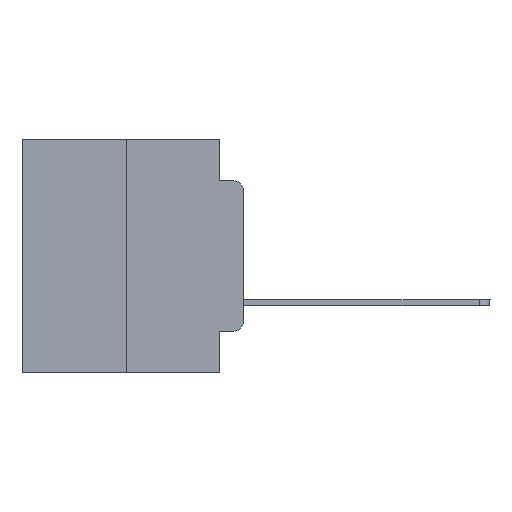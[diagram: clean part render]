
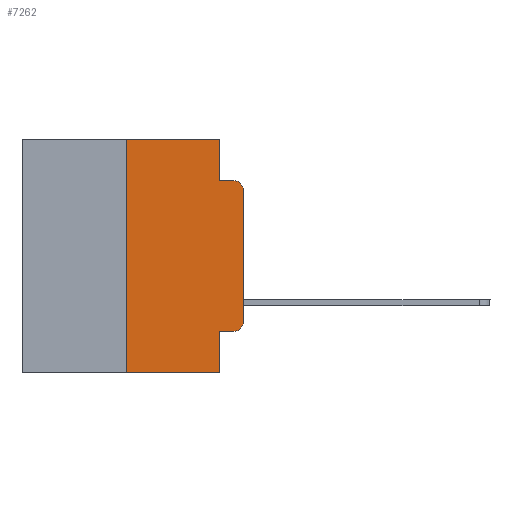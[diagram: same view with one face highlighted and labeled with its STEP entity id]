
A CAD part, left-side view. The second image highlights one B-rep face of the part: STEP entity #7262.
In plain terms, the highlighted planar face has unit normal (-1, 0, 0).
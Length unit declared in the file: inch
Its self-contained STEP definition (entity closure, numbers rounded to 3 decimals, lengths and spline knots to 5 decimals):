
#54 = LINE ( 'NONE', #8005, #21937 ) ;
#151 = CARTESIAN_POINT ( 'NONE',  ( 0., 0.02, -0.4115 ) ) ;
#272 = LINE ( 'NONE', #13980, #5402 ) ;
#963 = EDGE_CURVE ( 'NONE', #24113, #17036, #7960, .T. ) ;
#1355 = FACE_OUTER_BOUND ( 'NONE', #11826, .T. ) ;
#1591 = CARTESIAN_POINT ( 'NONE',  ( 0., 0.02, -0.0885 ) ) ;
#1706 = VECTOR ( 'NONE', #5119, 39.37008 ) ;
#1887 = CARTESIAN_POINT ( 'NONE',  ( 0., 0.25, 0. ) ) ;
#2122 = AXIS2_PLACEMENT_3D ( 'NONE', #11537, #19460, #17276 ) ;
#2824 = EDGE_CURVE ( 'NONE', #17036, #20742, #11524, .T. ) ;
#2998 = DIRECTION ( 'NONE',  ( 0., 0., -1. ) ) ;
#3121 = CARTESIAN_POINT ( 'NONE',  ( 0., 0.051, 0. ) ) ;
#3213 = VERTEX_POINT ( 'NONE', #18756 ) ;
#3263 = VERTEX_POINT ( 'NONE', #11593 ) ;
#3569 = PLANE ( 'NONE',  #2122 ) ;
#3600 = AXIS2_PLACEMENT_3D ( 'NONE', #15680, #3909, #11621 ) ;
#3909 = DIRECTION ( 'NONE',  ( -1., 0., 0. ) ) ;
#4227 = DIRECTION ( 'NONE',  ( 0., 0., -1. ) ) ;
#4660 = ORIENTED_EDGE ( 'NONE', *, *, #24435, .F. ) ;
#4749 = LINE ( 'NONE', #20508, #1706 ) ;
#4860 = ORIENTED_EDGE ( 'NONE', *, *, #963, .T. ) ;
#5119 = DIRECTION ( 'NONE',  ( 0., -1., 0. ) ) ;
#5402 = VECTOR ( 'NONE', #21869, 39.37008 ) ;
#5819 = EDGE_CURVE ( 'NONE', #13149, #12409, #4749, .T. ) ;
#6315 = ORIENTED_EDGE ( 'NONE', *, *, #11734, .F. ) ;
#6519 = EDGE_CURVE ( 'NONE', #13149, #14056, #272, .T. ) ;
#6989 = CARTESIAN_POINT ( 'NONE',  ( 0., 0.051, -0.0885 ) ) ;
#7262 = ADVANCED_FACE ( 'NONE', ( #1355 ), #3569, .F. ) ;
#7497 = ORIENTED_EDGE ( 'NONE', *, *, #25428, .T. ) ;
#7960 = LINE ( 'NONE', #9929, #23272 ) ;
#8005 = CARTESIAN_POINT ( 'NONE',  ( 0., 0., 0. ) ) ;
#8310 = ORIENTED_EDGE ( 'NONE', *, *, #6519, .F. ) ;
#8533 = CIRCLE ( 'NONE', #21038, 0.02 ) ;
#9397 = CARTESIAN_POINT ( 'NONE',  ( 0., 0.25, -0.5 ) ) ;
#9672 = DIRECTION ( 'NONE',  ( 0., 0., -1. ) ) ;
#9699 = VECTOR ( 'NONE', #24784, 39.37008 ) ;
#9929 = CARTESIAN_POINT ( 'NONE',  ( 0., 0.051, -0.4115 ) ) ;
#9946 = CARTESIAN_POINT ( 'NONE',  ( 0., 0., -0.1085 ) ) ;
#11093 = LINE ( 'NONE', #3121, #19722 ) ;
#11372 = VERTEX_POINT ( 'NONE', #1591 ) ;
#11524 = CIRCLE ( 'NONE', #3600, 0.02 ) ;
#11537 = CARTESIAN_POINT ( 'NONE',  ( 0., 0.473, 0. ) ) ;
#11593 = CARTESIAN_POINT ( 'NONE',  ( 0., 0.051, -0.0885 ) ) ;
#11621 = DIRECTION ( 'NONE',  ( 0., 0., -1. ) ) ;
#11689 = CARTESIAN_POINT ( 'NONE',  ( 0., 0.02, -0.1085 ) ) ;
#11734 = EDGE_CURVE ( 'NONE', #3213, #3263, #11093, .T. ) ;
#11826 = EDGE_LOOP ( 'NONE', ( #12894, #7497, #13380, #6315, #18050, #8310, #15507, #4660, #4860, #23856 ) ) ;
#11894 = VECTOR ( 'NONE', #22389, 39.37008 ) ;
#12409 = VERTEX_POINT ( 'NONE', #19884 ) ;
#12867 = EDGE_CURVE ( 'NONE', #14056, #3213, #24199, .T. ) ;
#12894 = ORIENTED_EDGE ( 'NONE', *, *, #15454, .T. ) ;
#13149 = VERTEX_POINT ( 'NONE', #9397 ) ;
#13380 = ORIENTED_EDGE ( 'NONE', *, *, #22109, .F. ) ;
#13848 = CARTESIAN_POINT ( 'NONE',  ( 0., 0.051, 0. ) ) ;
#13980 = CARTESIAN_POINT ( 'NONE',  ( 0., 0.25, 0. ) ) ;
#14056 = VERTEX_POINT ( 'NONE', #1887 ) ;
#14637 = CARTESIAN_POINT ( 'NONE',  ( 0., 0.473, 0. ) ) ;
#15454 = EDGE_CURVE ( 'NONE', #20742, #15766, #54, .T. ) ;
#15507 = ORIENTED_EDGE ( 'NONE', *, *, #5819, .T. ) ;
#15680 = CARTESIAN_POINT ( 'NONE',  ( 0., 0.02, -0.3915 ) ) ;
#15766 = VERTEX_POINT ( 'NONE', #9946 ) ;
#15978 = DIRECTION ( 'NONE',  ( 0., 0., 1. ) ) ;
#16346 = CARTESIAN_POINT ( 'NONE',  ( 0., 0.051, -0.4115 ) ) ;
#17036 = VERTEX_POINT ( 'NONE', #151 ) ;
#17096 = CARTESIAN_POINT ( 'NONE',  ( 0., 0., -0.3915 ) ) ;
#17276 = DIRECTION ( 'NONE',  ( 0., 0., -1. ) ) ;
#18050 = ORIENTED_EDGE ( 'NONE', *, *, #12867, .F. ) ;
#18756 = CARTESIAN_POINT ( 'NONE',  ( 0., 0.051, 0. ) ) ;
#19460 = DIRECTION ( 'NONE',  ( 1., 0., 0. ) ) ;
#19722 = VECTOR ( 'NONE', #2998, 39.37008 ) ;
#19873 = DIRECTION ( 'NONE',  ( -1., 0., 0. ) ) ;
#19884 = CARTESIAN_POINT ( 'NONE',  ( 0., 0.051, -0.5 ) ) ;
#20508 = CARTESIAN_POINT ( 'NONE',  ( 0., 0.473, -0.5 ) ) ;
#20742 = VERTEX_POINT ( 'NONE', #17096 ) ;
#21038 = AXIS2_PLACEMENT_3D ( 'NONE', #11689, #19873, #4227 ) ;
#21233 = LINE ( 'NONE', #13848, #22637 ) ;
#21869 = DIRECTION ( 'NONE',  ( 0., 0., 1. ) ) ;
#21937 = VECTOR ( 'NONE', #15978, 39.37008 ) ;
#22109 = EDGE_CURVE ( 'NONE', #3263, #11372, #24661, .T. ) ;
#22389 = DIRECTION ( 'NONE',  ( 0., -1., 0. ) ) ;
#22637 = VECTOR ( 'NONE', #9672, 39.37008 ) ;
#23272 = VECTOR ( 'NONE', #24183, 39.37008 ) ;
#23856 = ORIENTED_EDGE ( 'NONE', *, *, #2824, .T. ) ;
#24113 = VERTEX_POINT ( 'NONE', #16346 ) ;
#24183 = DIRECTION ( 'NONE',  ( 0., -1., 0. ) ) ;
#24199 = LINE ( 'NONE', #14637, #11894 ) ;
#24435 = EDGE_CURVE ( 'NONE', #24113, #12409, #21233, .T. ) ;
#24661 = LINE ( 'NONE', #6989, #9699 ) ;
#24784 = DIRECTION ( 'NONE',  ( 0., -1., 0. ) ) ;
#25428 = EDGE_CURVE ( 'NONE', #15766, #11372, #8533, .T. ) ;
